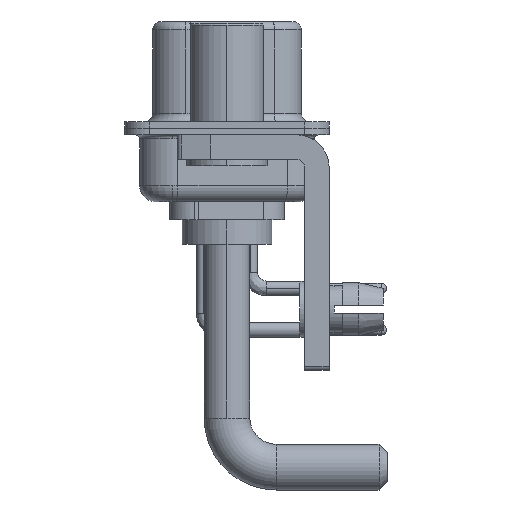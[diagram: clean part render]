
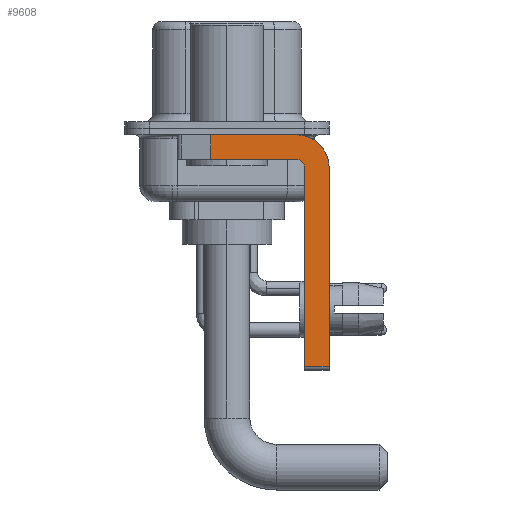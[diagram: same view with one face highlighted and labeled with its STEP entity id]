
A CAD part, left-side view. The second image highlights one B-rep face of the part: STEP entity #9608.
In plain terms, the highlighted planar face has unit normal (-1, 0, 0).
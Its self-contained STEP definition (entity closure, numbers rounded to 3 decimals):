
#154 = VECTOR ( 'NONE', #8574, 1000. ) ;
#970 = DIRECTION ( 'NONE',  ( 0., 0., -1. ) ) ;
#1009 = DIRECTION ( 'NONE',  ( 0., 0., -1. ) ) ;
#1332 = DIRECTION ( 'NONE',  ( -1., 0., 0. ) ) ;
#1496 = AXIS2_PLACEMENT_3D ( 'NONE', #8099, #1332, #16967 ) ;
#2228 = DIRECTION ( 'NONE',  ( 0., 0., -1. ) ) ;
#2373 = LINE ( 'NONE', #22139, #26895 ) ;
#2383 = CARTESIAN_POINT ( 'NONE',  ( -2.9, -6.25, -2.4 ) ) ;
#2542 = EDGE_CURVE ( 'NONE', #6689, #6543, #19014, .T. ) ;
#3179 = DIRECTION ( 'NONE',  ( 1., 0., 0. ) ) ;
#3475 = CARTESIAN_POINT ( 'NONE',  ( -2.9, 0.978, -1.9 ) ) ;
#4065 = CARTESIAN_POINT ( 'NONE',  ( -2.9, -4.25, -0.4 ) ) ;
#4373 = VECTOR ( 'NONE', #1009, 1000. ) ;
#6543 = VERTEX_POINT ( 'NONE', #4065 ) ;
#6689 = VERTEX_POINT ( 'NONE', #18656 ) ;
#6696 = LINE ( 'NONE', #20411, #25202 ) ;
#6832 = ORIENTED_EDGE ( 'NONE', *, *, #25166, .T. ) ;
#6864 = ORIENTED_EDGE ( 'NONE', *, *, #2542, .F. ) ;
#7213 = ORIENTED_EDGE ( 'NONE', *, *, #17825, .F. ) ;
#7623 = CIRCLE ( 'NONE', #1496, 0.5 ) ;
#8099 = CARTESIAN_POINT ( 'NONE',  ( -2.9, -4.25, -2.4 ) ) ;
#8365 = CARTESIAN_POINT ( 'NONE',  ( -2.9, 3., -0.4 ) ) ;
#8509 = VERTEX_POINT ( 'NONE', #22917 ) ;
#8574 = DIRECTION ( 'NONE',  ( 0., 1., 0. ) ) ;
#8801 = AXIS2_PLACEMENT_3D ( 'NONE', #24066, #3179, #970 ) ;
#8934 = ORIENTED_EDGE ( 'NONE', *, *, #21223, .F. ) ;
#9315 = CARTESIAN_POINT ( 'NONE',  ( -2.9, -4.25, -2.4 ) ) ;
#9608 = ADVANCED_FACE ( 'NONE', ( #18666 ), #19496, .F. ) ;
#10787 = CARTESIAN_POINT ( 'NONE',  ( -2.9, -4.25, -1.9 ) ) ;
#11035 = VERTEX_POINT ( 'NONE', #3475 ) ;
#11156 = CARTESIAN_POINT ( 'NONE',  ( -2.9, -4.75, -2.4 ) ) ;
#11688 = EDGE_LOOP ( 'NONE', ( #6864, #21277, #7213, #28560, #11874, #6832, #8934, #21921 ) ) ;
#11874 = ORIENTED_EDGE ( 'NONE', *, *, #13315, .F. ) ;
#12133 = VECTOR ( 'NONE', #20947, 1000. ) ;
#12356 = CIRCLE ( 'NONE', #13771, 2. ) ;
#13244 = VERTEX_POINT ( 'NONE', #25840 ) ;
#13315 = EDGE_CURVE ( 'NONE', #14771, #18781, #2373, .T. ) ;
#13771 = AXIS2_PLACEMENT_3D ( 'NONE', #9315, #22436, #2228 ) ;
#14696 = EDGE_CURVE ( 'NONE', #6543, #8509, #12356, .T. ) ;
#14771 = VERTEX_POINT ( 'NONE', #25241 ) ;
#14847 = EDGE_CURVE ( 'NONE', #18781, #13244, #7623, .T. ) ;
#15395 = DIRECTION ( 'NONE',  ( 0., -1., 0. ) ) ;
#16967 = DIRECTION ( 'NONE',  ( 0., 0., 1. ) ) ;
#17825 = EDGE_CURVE ( 'NONE', #13244, #11035, #22005, .T. ) ;
#18656 = CARTESIAN_POINT ( 'NONE',  ( -2.9, 0.978, -0.4 ) ) ;
#18666 = FACE_OUTER_BOUND ( 'NONE', #11688, .T. ) ;
#18781 = VERTEX_POINT ( 'NONE', #11156 ) ;
#19014 = LINE ( 'NONE', #8365, #25466 ) ;
#19496 = PLANE ( 'NONE',  #8801 ) ;
#20411 = CARTESIAN_POINT ( 'NONE',  ( -2.9, -4.25, -14.55 ) ) ;
#20947 = DIRECTION ( 'NONE',  ( 0., 0., -1. ) ) ;
#21223 = EDGE_CURVE ( 'NONE', #8509, #28860, #27184, .T. ) ;
#21277 = ORIENTED_EDGE ( 'NONE', *, *, #28808, .T. ) ;
#21921 = ORIENTED_EDGE ( 'NONE', *, *, #14696, .F. ) ;
#22005 = LINE ( 'NONE', #10787, #154 ) ;
#22139 = CARTESIAN_POINT ( 'NONE',  ( -2.9, -4.75, -14.8 ) ) ;
#22436 = DIRECTION ( 'NONE',  ( 1., 0., 0. ) ) ;
#22917 = CARTESIAN_POINT ( 'NONE',  ( -2.9, -6.25, -2.4 ) ) ;
#24066 = CARTESIAN_POINT ( 'NONE',  ( -2.9, -4.25, -2.4 ) ) ;
#24951 = DIRECTION ( 'NONE',  ( 0., 0., 1. ) ) ;
#25166 = EDGE_CURVE ( 'NONE', #14771, #28860, #6696, .T. ) ;
#25202 = VECTOR ( 'NONE', #15395, 1000. ) ;
#25229 = LINE ( 'NONE', #27745, #12133 ) ;
#25241 = CARTESIAN_POINT ( 'NONE',  ( -2.9, -4.75, -14.55 ) ) ;
#25466 = VECTOR ( 'NONE', #28590, 1000. ) ;
#25840 = CARTESIAN_POINT ( 'NONE',  ( -2.9, -4.25, -1.9 ) ) ;
#26240 = CARTESIAN_POINT ( 'NONE',  ( -2.9, -6.25, -14.55 ) ) ;
#26895 = VECTOR ( 'NONE', #24951, 1000. ) ;
#27184 = LINE ( 'NONE', #2383, #4373 ) ;
#27745 = CARTESIAN_POINT ( 'NONE',  ( -2.9, 0.978, -1.9 ) ) ;
#28560 = ORIENTED_EDGE ( 'NONE', *, *, #14847, .F. ) ;
#28590 = DIRECTION ( 'NONE',  ( 0., -1., 0. ) ) ;
#28808 = EDGE_CURVE ( 'NONE', #6689, #11035, #25229, .T. ) ;
#28860 = VERTEX_POINT ( 'NONE', #26240 ) ;
